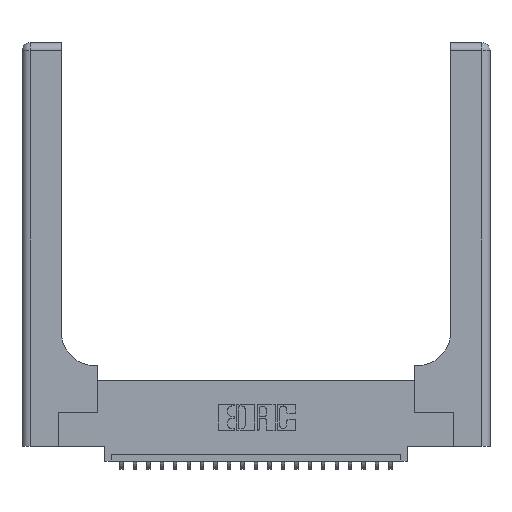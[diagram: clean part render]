
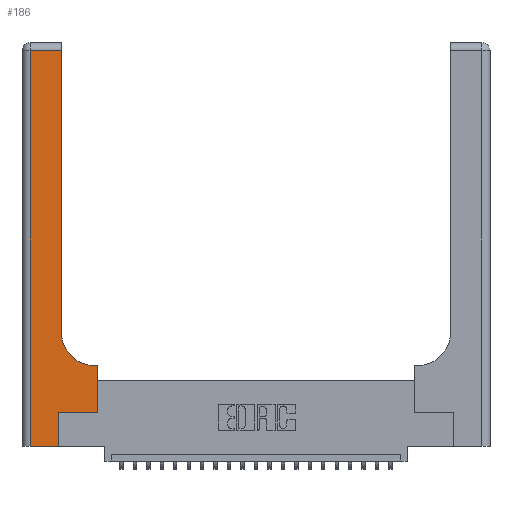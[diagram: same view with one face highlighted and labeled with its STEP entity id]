
A CAD part, top view. The second image highlights one B-rep face of the part: STEP entity #186.
In plain terms, the highlighted planar face has unit normal (0, 0, 1).
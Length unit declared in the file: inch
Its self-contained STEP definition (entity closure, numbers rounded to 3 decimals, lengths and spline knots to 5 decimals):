
#186 = ADVANCED_FACE ( 'NONE', ( #19979 ), #11953, .F. ) ;
#852 = DIRECTION ( 'NONE',  ( 0., 1., 0. ) ) ;
#1375 = VECTOR ( 'NONE', #23762, 39.37008 ) ;
#1500 = VERTEX_POINT ( 'NONE', #19795 ) ;
#1618 = CARTESIAN_POINT ( 'NONE',  ( 0.2915, 3., 0.37 ) ) ;
#1804 = CARTESIAN_POINT ( 'NONE',  ( 0.2915, 2.94, 0.37 ) ) ;
#2554 = LINE ( 'NONE', #3279, #15913 ) ;
#3055 = EDGE_CURVE ( 'NONE', #10714, #1500, #8912, .T. ) ;
#3279 = CARTESIAN_POINT ( 'NONE',  ( 0.269, 0.25, 0.37 ) ) ;
#3739 = ORIENTED_EDGE ( 'NONE', *, *, #20995, .T. ) ;
#4529 = DIRECTION ( 'NONE',  ( 0., -1., 0. ) ) ;
#4842 = VECTOR ( 'NONE', #4529, 39.37008 ) ;
#5137 = EDGE_CURVE ( 'NONE', #14194, #10001, #10519, .T. ) ;
#5485 = CARTESIAN_POINT ( 'NONE',  ( 0.5585, 0.6, 0.37 ) ) ;
#5552 = CARTESIAN_POINT ( 'NONE',  ( 0.5585, 0.25, 0.37 ) ) ;
#5555 = CARTESIAN_POINT ( 'NONE',  ( 0.5415, 0.6, 0.37 ) ) ;
#5804 = CARTESIAN_POINT ( 'NONE',  ( 0.5415, 0.85, 0.37 ) ) ;
#6554 = CARTESIAN_POINT ( 'NONE',  ( 0., 3., 0.37 ) ) ;
#6775 = CARTESIAN_POINT ( 'NONE',  ( 0.06, 0., 0.37 ) ) ;
#7062 = VECTOR ( 'NONE', #8110, 39.37008 ) ;
#8097 = LINE ( 'NONE', #1618, #1375 ) ;
#8110 = DIRECTION ( 'NONE',  ( -1., 0., 0. ) ) ;
#8527 = EDGE_CURVE ( 'NONE', #22005, #10714, #16746, .T. ) ;
#8661 = DIRECTION ( 'NONE',  ( 0., 0., -1. ) ) ;
#8912 = LINE ( 'NONE', #23067, #12666 ) ;
#9232 = ORIENTED_EDGE ( 'NONE', *, *, #21844, .T. ) ;
#9533 = VERTEX_POINT ( 'NONE', #1804 ) ;
#10001 = VERTEX_POINT ( 'NONE', #5485 ) ;
#10403 = EDGE_CURVE ( 'NONE', #9533, #13249, #12537, .T. ) ;
#10519 = LINE ( 'NONE', #5552, #13408 ) ;
#10714 = VERTEX_POINT ( 'NONE', #19986 ) ;
#10830 = DIRECTION ( 'NONE',  ( 1., 0., 0. ) ) ;
#11131 = DIRECTION ( 'NONE',  ( 0., 1., 0. ) ) ;
#11953 = PLANE ( 'NONE',  #21619 ) ;
#12537 = LINE ( 'NONE', #18729, #13363 ) ;
#12666 = VECTOR ( 'NONE', #852, 39.37008 ) ;
#12875 = CARTESIAN_POINT ( 'NONE',  ( 0.06, 2.94, 0.37 ) ) ;
#12981 = ORIENTED_EDGE ( 'NONE', *, *, #3055, .T. ) ;
#13249 = VERTEX_POINT ( 'NONE', #12875 ) ;
#13363 = VECTOR ( 'NONE', #20580, 39.37008 ) ;
#13408 = VECTOR ( 'NONE', #11131, 39.37008 ) ;
#13543 = CARTESIAN_POINT ( 'NONE',  ( 0.5585, 0.25, 0.37 ) ) ;
#14194 = VERTEX_POINT ( 'NONE', #13543 ) ;
#15787 = ORIENTED_EDGE ( 'NONE', *, *, #5137, .T. ) ;
#15839 = DIRECTION ( 'NONE',  ( -1., 0., 0. ) ) ;
#15913 = VECTOR ( 'NONE', #10830, 39.37008 ) ;
#16536 = AXIS2_PLACEMENT_3D ( 'NONE', #5804, #18750, #22226 ) ;
#16746 = LINE ( 'NONE', #20560, #19907 ) ;
#17236 = ORIENTED_EDGE ( 'NONE', *, *, #19126, .T. ) ;
#17917 = EDGE_LOOP ( 'NONE', ( #3739, #23977, #9232, #20066, #12981, #23702, #15787, #17236, #18868 ) ) ;
#18299 = CIRCLE ( 'NONE', #16536, 0.25 ) ;
#18729 = CARTESIAN_POINT ( 'NONE',  ( 0., 2.94, 0.37 ) ) ;
#18750 = DIRECTION ( 'NONE',  ( 0., 0., -1. ) ) ;
#18868 = ORIENTED_EDGE ( 'NONE', *, *, #19549, .T. ) ;
#19126 = EDGE_CURVE ( 'NONE', #10001, #23175, #21788, .T. ) ;
#19549 = EDGE_CURVE ( 'NONE', #23175, #21037, #18299, .T. ) ;
#19795 = CARTESIAN_POINT ( 'NONE',  ( 0.269, 0.25, 0.37 ) ) ;
#19907 = VECTOR ( 'NONE', #22264, 39.37008 ) ;
#19979 = FACE_OUTER_BOUND ( 'NONE', #17917, .T. ) ;
#19986 = CARTESIAN_POINT ( 'NONE',  ( 0.269, 0., 0.37 ) ) ;
#20066 = ORIENTED_EDGE ( 'NONE', *, *, #8527, .T. ) ;
#20176 = LINE ( 'NONE', #23324, #4842 ) ;
#20189 = CARTESIAN_POINT ( 'NONE',  ( 0.2915, 0.85, 0.37 ) ) ;
#20560 = CARTESIAN_POINT ( 'NONE',  ( 0., 0., 0.37 ) ) ;
#20580 = DIRECTION ( 'NONE',  ( -1., 0., 0. ) ) ;
#20921 = EDGE_CURVE ( 'NONE', #1500, #14194, #2554, .T. ) ;
#20995 = EDGE_CURVE ( 'NONE', #21037, #9533, #8097, .T. ) ;
#21037 = VERTEX_POINT ( 'NONE', #20189 ) ;
#21619 = AXIS2_PLACEMENT_3D ( 'NONE', #6554, #8661, #15839 ) ;
#21788 = LINE ( 'NONE', #23137, #7062 ) ;
#21844 = EDGE_CURVE ( 'NONE', #13249, #22005, #20176, .T. ) ;
#22005 = VERTEX_POINT ( 'NONE', #6775 ) ;
#22226 = DIRECTION ( 'NONE',  ( 1., 0., 0. ) ) ;
#22264 = DIRECTION ( 'NONE',  ( 1., 0., 0. ) ) ;
#23067 = CARTESIAN_POINT ( 'NONE',  ( 0.269, 0., 0.37 ) ) ;
#23137 = CARTESIAN_POINT ( 'NONE',  ( 0.2915, 0.6, 0.37 ) ) ;
#23175 = VERTEX_POINT ( 'NONE', #5555 ) ;
#23324 = CARTESIAN_POINT ( 'NONE',  ( 0.06, 3., 0.37 ) ) ;
#23702 = ORIENTED_EDGE ( 'NONE', *, *, #20921, .T. ) ;
#23762 = DIRECTION ( 'NONE',  ( 0., 1., 0. ) ) ;
#23977 = ORIENTED_EDGE ( 'NONE', *, *, #10403, .T. ) ;
